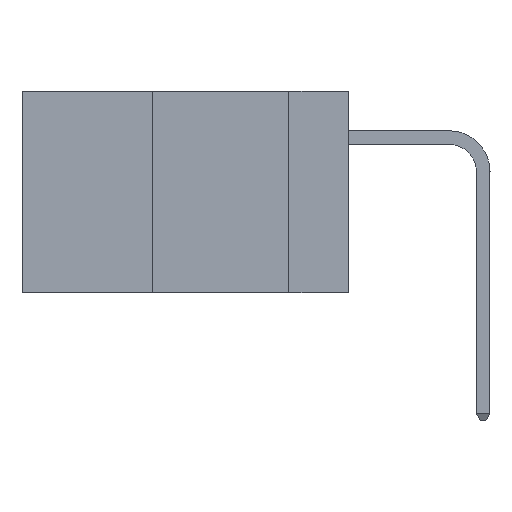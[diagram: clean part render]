
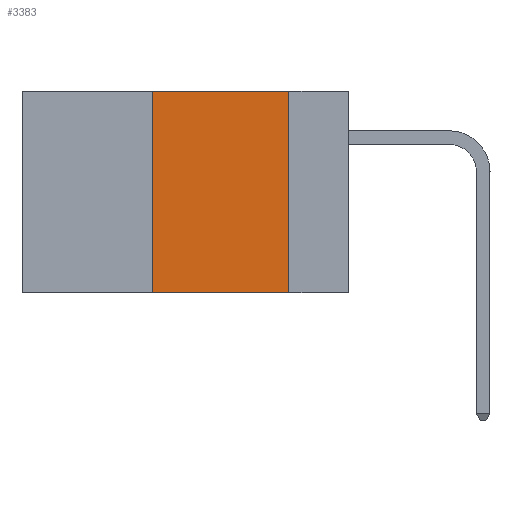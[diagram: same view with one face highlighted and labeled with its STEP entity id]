
A CAD part, left-side view. The second image highlights one B-rep face of the part: STEP entity #3383.
In plain terms, the highlighted planar face has unit normal (-1, 0, 0).
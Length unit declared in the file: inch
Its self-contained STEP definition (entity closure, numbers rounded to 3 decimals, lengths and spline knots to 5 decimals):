
#1319 = VECTOR ( 'NONE', #6504, 39.37008 ) ;
#1783 = EDGE_LOOP ( 'NONE', ( #7825, #13018, #8122, #13797 ) ) ;
#3383 = ADVANCED_FACE ( 'NONE', ( #7774 ), #15662, .F. ) ;
#3508 = CARTESIAN_POINT ( 'NONE',  ( 0., 0.36, 0. ) ) ;
#4076 = DIRECTION ( 'NONE',  ( 1., 0., 0. ) ) ;
#4392 = CARTESIAN_POINT ( 'NONE',  ( 0., 0.11, -0.37 ) ) ;
#4596 = CARTESIAN_POINT ( 'NONE',  ( 0., 0.11, 0. ) ) ;
#4798 = DIRECTION ( 'NONE',  ( 0., 0., 1. ) ) ;
#4825 = LINE ( 'NONE', #10072, #11118 ) ;
#5110 = VERTEX_POINT ( 'NONE', #4596 ) ;
#5982 = EDGE_CURVE ( 'NONE', #5110, #8874, #4825, .T. ) ;
#6504 = DIRECTION ( 'NONE',  ( 0., -1., 0. ) ) ;
#7774 = FACE_OUTER_BOUND ( 'NONE', #1783, .T. ) ;
#7825 = ORIENTED_EDGE ( 'NONE', *, *, #5982, .F. ) ;
#8122 = ORIENTED_EDGE ( 'NONE', *, *, #8450, .F. ) ;
#8206 = LINE ( 'NONE', #12555, #1319 ) ;
#8450 = EDGE_CURVE ( 'NONE', #8723, #12457, #8991, .T. ) ;
#8548 = VECTOR ( 'NONE', #14196, 39.37008 ) ;
#8723 = VERTEX_POINT ( 'NONE', #12702 ) ;
#8874 = VERTEX_POINT ( 'NONE', #4392 ) ;
#8929 = LINE ( 'NONE', #11959, #8548 ) ;
#8991 = LINE ( 'NONE', #3508, #14732 ) ;
#9258 = CARTESIAN_POINT ( 'NONE',  ( 0., 0.6, 0. ) ) ;
#9359 = DIRECTION ( 'NONE',  ( 0., 0., -1. ) ) ;
#10072 = CARTESIAN_POINT ( 'NONE',  ( 0., 0.11, 0. ) ) ;
#10239 = EDGE_CURVE ( 'NONE', #8723, #8874, #8929, .T. ) ;
#11118 = VECTOR ( 'NONE', #11802, 39.37008 ) ;
#11309 = AXIS2_PLACEMENT_3D ( 'NONE', #9258, #4076, #9359 ) ;
#11802 = DIRECTION ( 'NONE',  ( 0., 0., -1. ) ) ;
#11959 = CARTESIAN_POINT ( 'NONE',  ( 0., 0.6, -0.37 ) ) ;
#12259 = CARTESIAN_POINT ( 'NONE',  ( 0., 0.36, 0. ) ) ;
#12457 = VERTEX_POINT ( 'NONE', #12259 ) ;
#12555 = CARTESIAN_POINT ( 'NONE',  ( 0., 0.6, 0. ) ) ;
#12702 = CARTESIAN_POINT ( 'NONE',  ( 0., 0.36, -0.37 ) ) ;
#13018 = ORIENTED_EDGE ( 'NONE', *, *, #14121, .F. ) ;
#13797 = ORIENTED_EDGE ( 'NONE', *, *, #10239, .T. ) ;
#14121 = EDGE_CURVE ( 'NONE', #12457, #5110, #8206, .T. ) ;
#14196 = DIRECTION ( 'NONE',  ( 0., -1., 0. ) ) ;
#14732 = VECTOR ( 'NONE', #4798, 39.37008 ) ;
#15662 = PLANE ( 'NONE',  #11309 ) ;
